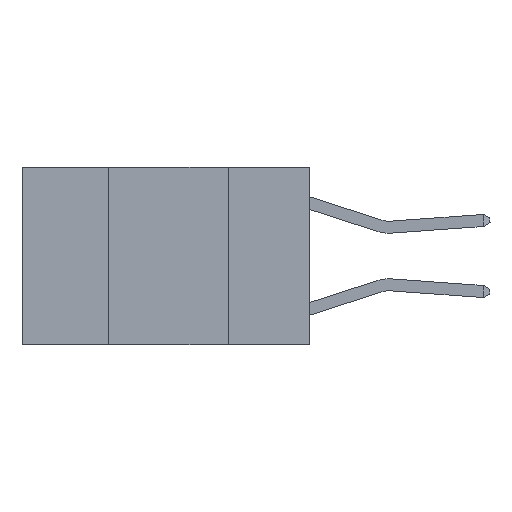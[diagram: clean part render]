
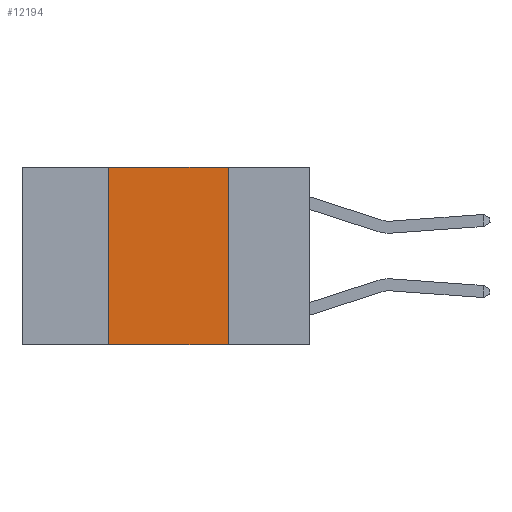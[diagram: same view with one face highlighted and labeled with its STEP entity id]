
A CAD part, left-side view. The second image highlights one B-rep face of the part: STEP entity #12194.
In plain terms, the highlighted planar face has unit normal (-1, 0, 0).
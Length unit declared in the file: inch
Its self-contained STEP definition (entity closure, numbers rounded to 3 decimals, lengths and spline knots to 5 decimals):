
#203 = CARTESIAN_POINT ( 'NONE',  ( 0., 0.17, -0.37 ) ) ;
#222 = DIRECTION ( 'NONE',  ( 0., 0., -1. ) ) ;
#370 = VERTEX_POINT ( 'NONE', #6809 ) ;
#619 = EDGE_CURVE ( 'NONE', #2392, #370, #4122, .T. ) ;
#739 = ORIENTED_EDGE ( 'NONE', *, *, #11672, .F. ) ;
#1353 = ORIENTED_EDGE ( 'NONE', *, *, #7054, .T. ) ;
#1677 = CARTESIAN_POINT ( 'NONE',  ( 0., 0.6, -0.37 ) ) ;
#1716 = DIRECTION ( 'NONE',  ( 0., 0., -1. ) ) ;
#2216 = VERTEX_POINT ( 'NONE', #203 ) ;
#2266 = ORIENTED_EDGE ( 'NONE', *, *, #619, .F. ) ;
#2392 = VERTEX_POINT ( 'NONE', #9587 ) ;
#3713 = VECTOR ( 'NONE', #12442, 39.37008 ) ;
#3722 = VECTOR ( 'NONE', #8038, 39.37008 ) ;
#3847 = EDGE_CURVE ( 'NONE', #6240, #2216, #13856, .T. ) ;
#4122 = LINE ( 'NONE', #9666, #3713 ) ;
#4170 = VECTOR ( 'NONE', #222, 39.37008 ) ;
#4207 = CARTESIAN_POINT ( 'NONE',  ( 0., 0.6, 0. ) ) ;
#4719 = ORIENTED_EDGE ( 'NONE', *, *, #3847, .F. ) ;
#5291 = DIRECTION ( 'NONE',  ( 0., -1., 0. ) ) ;
#5773 = EDGE_LOOP ( 'NONE', ( #4719, #739, #2266, #1353 ) ) ;
#5811 = CARTESIAN_POINT ( 'NONE',  ( 0., 0.17, 0. ) ) ;
#6240 = VERTEX_POINT ( 'NONE', #5811 ) ;
#6809 = CARTESIAN_POINT ( 'NONE',  ( 0., 0.42, 0. ) ) ;
#7054 = EDGE_CURVE ( 'NONE', #2392, #2216, #7440, .T. ) ;
#7440 = LINE ( 'NONE', #1677, #3722 ) ;
#8038 = DIRECTION ( 'NONE',  ( 0., -1., 0. ) ) ;
#9024 = CARTESIAN_POINT ( 'NONE',  ( 0., 0.6, 0. ) ) ;
#9268 = DIRECTION ( 'NONE',  ( 1., 0., 0. ) ) ;
#9587 = CARTESIAN_POINT ( 'NONE',  ( 0., 0.42, -0.37 ) ) ;
#9666 = CARTESIAN_POINT ( 'NONE',  ( 0., 0.42, 0. ) ) ;
#10767 = AXIS2_PLACEMENT_3D ( 'NONE', #4207, #9268, #1716 ) ;
#11004 = VECTOR ( 'NONE', #5291, 39.37008 ) ;
#11375 = LINE ( 'NONE', #9024, #11004 ) ;
#11672 = EDGE_CURVE ( 'NONE', #370, #6240, #11375, .T. ) ;
#12194 = ADVANCED_FACE ( 'NONE', ( #15516 ), #13869, .F. ) ;
#12442 = DIRECTION ( 'NONE',  ( 0., 0., 1. ) ) ;
#12678 = CARTESIAN_POINT ( 'NONE',  ( 0., 0.17, 0. ) ) ;
#13856 = LINE ( 'NONE', #12678, #4170 ) ;
#13869 = PLANE ( 'NONE',  #10767 ) ;
#15516 = FACE_OUTER_BOUND ( 'NONE', #5773, .T. ) ;
